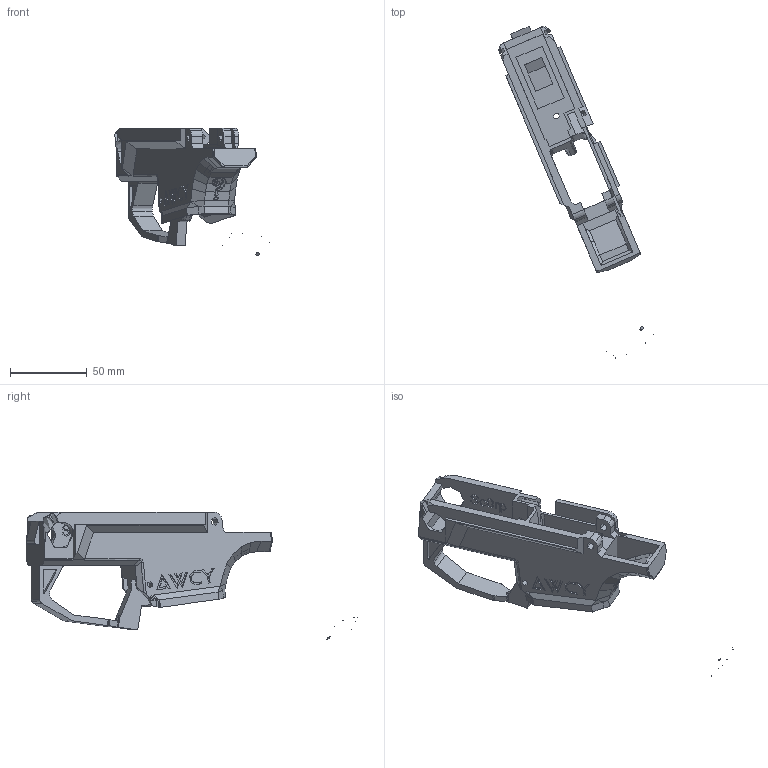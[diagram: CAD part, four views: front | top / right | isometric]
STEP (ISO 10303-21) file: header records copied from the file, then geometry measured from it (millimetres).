
FILE_DESCRIPTION(('STEP AP214'),'1');
FILE_NAME('ACWY Scorpion lower double signed with qmark.stp','2020-10-03T18:28:23',(' '),(' '),'Spatial InterOp 3D',' ',' ');
FILE_SCHEMA(('AUTOMOTIVE_DESIGN { 1 0 10303 214 1 1 1 1 }'));
Length unit declared in the file: metre
Products named in the file (5): ACWY Scorpion lower double signed with qmark; ACWY Scorpion lower signed; Final CZ Scorpion Lower v62 (1); CZ Scorpion evo lower v20 (2); Final CZ Scorpion LOWER ONLY v2 (1)
Assembly tree (4 placements, depth 4):
  ACWY Scorpion lower double signed with qmark
    ACWY Scorpion lower signed
    Final CZ Scorpion LOWER ONLY v2 (1)
      Final CZ Scorpion Lower v62 (1)
        CZ Scorpion evo lower v20 (2)
Bounding box: 100.66 x 215.61 x 82.71 mm (x, y, z)
Volume: 77784.5 mm3; surface area: 45237.9 mm2
Topology: 3 solids, 27 shells, 1394 faces, 4875 edges, 3874 vertices
Faces by surface type: plane 752, cylinder 361, extrusion 152, bspline 129
Entity records: 63072 total; most frequent: CARTESIAN_POINT 19780, ORIENTED_EDGE 8634, DIRECTION 7728, EDGE_CURVE 4512, VECTOR 3242, VERTEX_POINT 3171, LINE 3090, AXIS2_PLACEMENT_3D 2243
